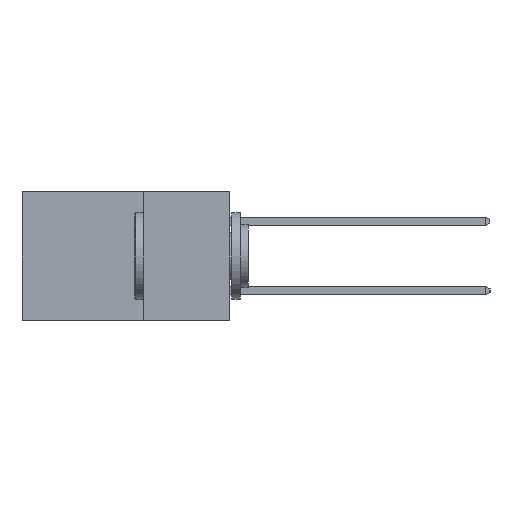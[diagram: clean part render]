
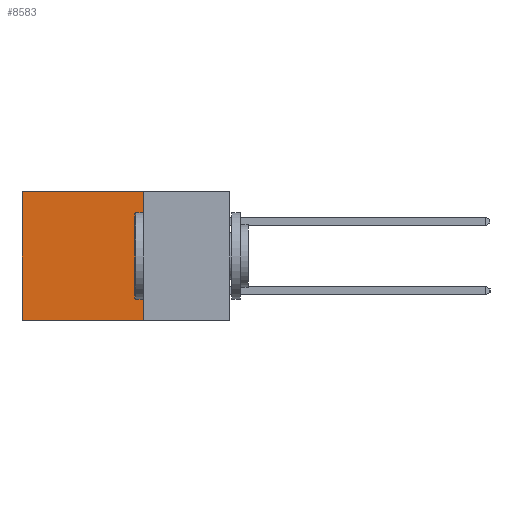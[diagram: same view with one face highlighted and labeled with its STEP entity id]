
A CAD part, left-side view. The second image highlights one B-rep face of the part: STEP entity #8583.
In plain terms, the highlighted planar face has unit normal (-1, 0, 0).
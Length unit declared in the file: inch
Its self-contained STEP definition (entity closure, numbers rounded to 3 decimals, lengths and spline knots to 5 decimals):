
#17 = DIRECTION ( 'NONE',  ( 0., 1., 0. ) ) ;
#179 = LINE ( 'NONE', #4568, #12699 ) ;
#510 = LINE ( 'NONE', #10309, #7103 ) ;
#725 = AXIS2_PLACEMENT_3D ( 'NONE', #2881, #2986, #2791 ) ;
#1466 = CARTESIAN_POINT ( 'NONE',  ( 0.2615, 0.6, -0.37 ) ) ;
#1600 = DIRECTION ( 'NONE',  ( 0., 0., -1. ) ) ;
#1624 = EDGE_LOOP ( 'NONE', ( #13517, #3050, #11318, #4478 ) ) ;
#2292 = CARTESIAN_POINT ( 'NONE',  ( 0.2615, 0.25, -0.37 ) ) ;
#2791 = DIRECTION ( 'NONE',  ( 0., 0., -1. ) ) ;
#2881 = CARTESIAN_POINT ( 'NONE',  ( 0.2615, 0.25, -0.37 ) ) ;
#2902 = LINE ( 'NONE', #4706, #5968 ) ;
#2986 = DIRECTION ( 'NONE',  ( 1., 0., 0. ) ) ;
#3037 = CARTESIAN_POINT ( 'NONE',  ( 0.2615, 0.25, 0. ) ) ;
#3050 = ORIENTED_EDGE ( 'NONE', *, *, #5736, .F. ) ;
#3126 = PLANE ( 'NONE',  #725 ) ;
#3845 = DIRECTION ( 'NONE',  ( 0., 1., 0. ) ) ;
#4478 = ORIENTED_EDGE ( 'NONE', *, *, #5236, .T. ) ;
#4568 = CARTESIAN_POINT ( 'NONE',  ( 0.2615, 0.25, 0. ) ) ;
#4706 = CARTESIAN_POINT ( 'NONE',  ( 0.2615, 0.25, -0.37 ) ) ;
#4951 = VERTEX_POINT ( 'NONE', #12007 ) ;
#5236 = EDGE_CURVE ( 'NONE', #13356, #8713, #179, .T. ) ;
#5736 = EDGE_CURVE ( 'NONE', #6346, #4951, #2902, .T. ) ;
#5968 = VECTOR ( 'NONE', #17, 39.37008 ) ;
#6346 = VERTEX_POINT ( 'NONE', #2292 ) ;
#7103 = VECTOR ( 'NONE', #9180, 39.37008 ) ;
#7985 = LINE ( 'NONE', #1466, #15378 ) ;
#8583 = ADVANCED_FACE ( 'NONE', ( #9034 ), #3126, .F. ) ;
#8713 = VERTEX_POINT ( 'NONE', #16338 ) ;
#9034 = FACE_OUTER_BOUND ( 'NONE', #1624, .T. ) ;
#9180 = DIRECTION ( 'NONE',  ( 0., 0., -1. ) ) ;
#10309 = CARTESIAN_POINT ( 'NONE',  ( 0.2615, 0.25, -0.37 ) ) ;
#10450 = EDGE_CURVE ( 'NONE', #8713, #4951, #7985, .T. ) ;
#11318 = ORIENTED_EDGE ( 'NONE', *, *, #13888, .F. ) ;
#12007 = CARTESIAN_POINT ( 'NONE',  ( 0.2615, 0.6, -0.37 ) ) ;
#12699 = VECTOR ( 'NONE', #3845, 39.37008 ) ;
#13356 = VERTEX_POINT ( 'NONE', #3037 ) ;
#13517 = ORIENTED_EDGE ( 'NONE', *, *, #10450, .T. ) ;
#13888 = EDGE_CURVE ( 'NONE', #13356, #6346, #510, .T. ) ;
#15378 = VECTOR ( 'NONE', #1600, 39.37008 ) ;
#16338 = CARTESIAN_POINT ( 'NONE',  ( 0.2615, 0.6, 0. ) ) ;
